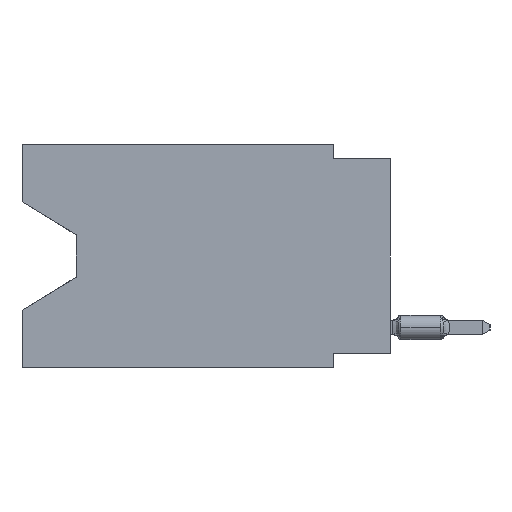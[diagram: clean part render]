
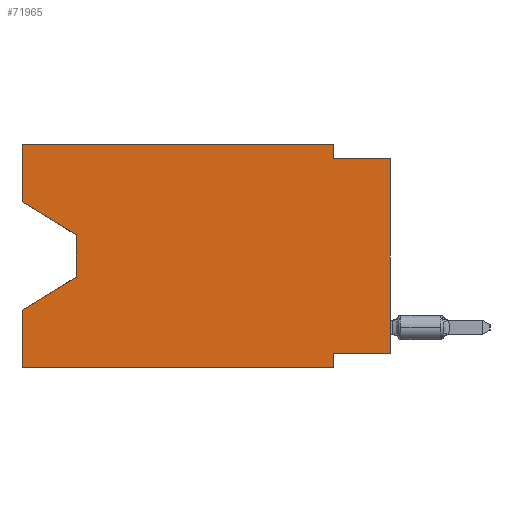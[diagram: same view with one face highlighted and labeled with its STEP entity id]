
A CAD part, left-side view. The second image highlights one B-rep face of the part: STEP entity #71965.
In plain terms, the highlighted planar face has unit normal (-1, 0, 0).
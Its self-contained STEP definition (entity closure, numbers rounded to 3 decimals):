
#1093 = VECTOR ( 'NONE', #67676, 1000. ) ;
#1139 = CARTESIAN_POINT ( 'NONE',  ( 0., 16.383, -2.546 ) ) ;
#1369 = CARTESIAN_POINT ( 'NONE',  ( 0., 13.97, -5.893 ) ) ;
#2217 = LINE ( 'NONE', #28104, #41991 ) ;
#2466 = VERTEX_POINT ( 'NONE', #38149 ) ;
#2677 = DIRECTION ( 'NONE',  ( 0., 0.855, -0.519 ) ) ;
#2856 = ORIENTED_EDGE ( 'NONE', *, *, #49656, .T. ) ;
#4470 = VECTOR ( 'NONE', #2677, 1000. ) ;
#5207 = ORIENTED_EDGE ( 'NONE', *, *, #22602, .T. ) ;
#5239 = ORIENTED_EDGE ( 'NONE', *, *, #23299, .T. ) ;
#5296 = LINE ( 'NONE', #37587, #50493 ) ;
#5646 = CARTESIAN_POINT ( 'NONE',  ( 0., 2.54, -9.906 ) ) ;
#7098 = FACE_OUTER_BOUND ( 'NONE', #19887, .T. ) ;
#7330 = EDGE_CURVE ( 'NONE', #18322, #49611, #44204, .T. ) ;
#7959 = VECTOR ( 'NONE', #17008, 1000. ) ;
#8356 = CARTESIAN_POINT ( 'NONE',  ( 0., 16.383, 0. ) ) ;
#10038 = CARTESIAN_POINT ( 'NONE',  ( 0., 0., -9.271 ) ) ;
#11566 = CARTESIAN_POINT ( 'NONE',  ( 0., 0., -9.271 ) ) ;
#11954 = ORIENTED_EDGE ( 'NONE', *, *, #74613, .F. ) ;
#13325 = EDGE_CURVE ( 'NONE', #49611, #65926, #22198, .T. ) ;
#13948 = CARTESIAN_POINT ( 'NONE',  ( 0., 0., -0.635 ) ) ;
#14406 = ORIENTED_EDGE ( 'NONE', *, *, #48312, .F. ) ;
#15111 = DIRECTION ( 'NONE',  ( 1., 0., 0. ) ) ;
#17008 = DIRECTION ( 'NONE',  ( 0., 0., -1. ) ) ;
#18322 = VERTEX_POINT ( 'NONE', #65536 ) ;
#19887 = EDGE_LOOP ( 'NONE', ( #5239, #55289, #66443, #54813, #5207, #72661, #11954, #2856, #14406, #29574, #67841, #52360 ) ) ;
#20196 = EDGE_CURVE ( 'NONE', #74292, #59708, #28682, .T. ) ;
#20670 = DIRECTION ( 'NONE',  ( 0., -0.855, -0.519 ) ) ;
#22198 = LINE ( 'NONE', #82122, #4470 ) ;
#22303 = DIRECTION ( 'NONE',  ( 0., 0., -1. ) ) ;
#22363 = DIRECTION ( 'NONE',  ( 0., 1., 0. ) ) ;
#22602 = EDGE_CURVE ( 'NONE', #61736, #59708, #33088, .T. ) ;
#23299 = EDGE_CURVE ( 'NONE', #57706, #18322, #39796, .T. ) ;
#24556 = VERTEX_POINT ( 'NONE', #13948 ) ;
#25495 = CARTESIAN_POINT ( 'NONE',  ( 0., 2.54, -9.271 ) ) ;
#26490 = DIRECTION ( 'NONE',  ( 0., -1., 0. ) ) ;
#28104 = CARTESIAN_POINT ( 'NONE',  ( 0., 0., 0. ) ) ;
#28682 = LINE ( 'NONE', #41010, #69854 ) ;
#29574 = ORIENTED_EDGE ( 'NONE', *, *, #31948, .F. ) ;
#31426 = CARTESIAN_POINT ( 'NONE',  ( 0., 13.97, -4.013 ) ) ;
#31948 = EDGE_CURVE ( 'NONE', #51112, #2466, #33709, .T. ) ;
#32020 = EDGE_CURVE ( 'NONE', #61736, #65926, #61739, .T. ) ;
#32816 = CARTESIAN_POINT ( 'NONE',  ( 0., 16.383, -2.546 ) ) ;
#33088 = LINE ( 'NONE', #46265, #62007 ) ;
#33709 = LINE ( 'NONE', #64355, #81165 ) ;
#37587 = CARTESIAN_POINT ( 'NONE',  ( 0., 16.383, 0. ) ) ;
#38065 = EDGE_CURVE ( 'NONE', #57706, #54220, #5296, .T. ) ;
#38149 = CARTESIAN_POINT ( 'NONE',  ( 0., 2.54, -0.635 ) ) ;
#38659 = AXIS2_PLACEMENT_3D ( 'NONE', #8356, #15111, #78914 ) ;
#39198 = CARTESIAN_POINT ( 'NONE',  ( 0., 16.383, -9.906 ) ) ;
#39708 = VECTOR ( 'NONE', #26490, 1000. ) ;
#39793 = PLANE ( 'NONE',  #38659 ) ;
#39796 = LINE ( 'NONE', #1139, #81090 ) ;
#41010 = CARTESIAN_POINT ( 'NONE',  ( 0., 2.54, -9.906 ) ) ;
#41991 = VECTOR ( 'NONE', #54022, 1000. ) ;
#42526 = CARTESIAN_POINT ( 'NONE',  ( 0., 2.54, 0. ) ) ;
#44204 = LINE ( 'NONE', #31426, #7959 ) ;
#44514 = VECTOR ( 'NONE', #22363, 1000. ) ;
#46265 = CARTESIAN_POINT ( 'NONE',  ( 0., 16.383, -9.906 ) ) ;
#46710 = DIRECTION ( 'NONE',  ( 0., -1., 0. ) ) ;
#46730 = VERTEX_POINT ( 'NONE', #11566 ) ;
#48312 = EDGE_CURVE ( 'NONE', #2466, #24556, #70215, .T. ) ;
#49611 = VERTEX_POINT ( 'NONE', #1369 ) ;
#49656 = EDGE_CURVE ( 'NONE', #46730, #24556, #2217, .T. ) ;
#50493 = VECTOR ( 'NONE', #83080, 1000. ) ;
#51112 = VERTEX_POINT ( 'NONE', #42526 ) ;
#52360 = ORIENTED_EDGE ( 'NONE', *, *, #38065, .F. ) ;
#52551 = CARTESIAN_POINT ( 'NONE',  ( 0., 16.383, -7.36 ) ) ;
#53819 = EDGE_CURVE ( 'NONE', #54220, #51112, #71531, .T. ) ;
#54022 = DIRECTION ( 'NONE',  ( 0., 0., 1. ) ) ;
#54220 = VERTEX_POINT ( 'NONE', #71437 ) ;
#54813 = ORIENTED_EDGE ( 'NONE', *, *, #32020, .F. ) ;
#55289 = ORIENTED_EDGE ( 'NONE', *, *, #7330, .T. ) ;
#55330 = CARTESIAN_POINT ( 'NONE',  ( 0., 16.383, 0. ) ) ;
#57706 = VERTEX_POINT ( 'NONE', #32816 ) ;
#57952 = DIRECTION ( 'NONE',  ( 0., 0., -1. ) ) ;
#58778 = CARTESIAN_POINT ( 'NONE',  ( 0., 16.383, 0. ) ) ;
#59025 = DIRECTION ( 'NONE',  ( 0., -1., 0. ) ) ;
#59708 = VERTEX_POINT ( 'NONE', #5646 ) ;
#61736 = VERTEX_POINT ( 'NONE', #39198 ) ;
#61739 = LINE ( 'NONE', #55330, #1093 ) ;
#62007 = VECTOR ( 'NONE', #59025, 1000. ) ;
#63838 = CARTESIAN_POINT ( 'NONE',  ( 0., 0., -0.635 ) ) ;
#64355 = CARTESIAN_POINT ( 'NONE',  ( 0., 2.54, 0. ) ) ;
#65536 = CARTESIAN_POINT ( 'NONE',  ( 0., 13.97, -4.013 ) ) ;
#65926 = VERTEX_POINT ( 'NONE', #52551 ) ;
#66443 = ORIENTED_EDGE ( 'NONE', *, *, #13325, .T. ) ;
#67676 = DIRECTION ( 'NONE',  ( 0., 0., 1. ) ) ;
#67841 = ORIENTED_EDGE ( 'NONE', *, *, #53819, .F. ) ;
#68249 = LINE ( 'NONE', #10038, #44514 ) ;
#69854 = VECTOR ( 'NONE', #22303, 1000. ) ;
#70215 = LINE ( 'NONE', #63838, #73280 ) ;
#71437 = CARTESIAN_POINT ( 'NONE',  ( 0., 16.383, 0. ) ) ;
#71531 = LINE ( 'NONE', #58778, #39708 ) ;
#71965 = ADVANCED_FACE ( 'NONE', ( #7098 ), #39793, .F. ) ;
#72661 = ORIENTED_EDGE ( 'NONE', *, *, #20196, .F. ) ;
#73280 = VECTOR ( 'NONE', #46710, 1000. ) ;
#74292 = VERTEX_POINT ( 'NONE', #25495 ) ;
#74613 = EDGE_CURVE ( 'NONE', #46730, #74292, #68249, .T. ) ;
#78914 = DIRECTION ( 'NONE',  ( 0., 0., -1. ) ) ;
#81090 = VECTOR ( 'NONE', #20670, 1000. ) ;
#81165 = VECTOR ( 'NONE', #57952, 1000. ) ;
#82122 = CARTESIAN_POINT ( 'NONE',  ( 0., 13.97, -5.893 ) ) ;
#83080 = DIRECTION ( 'NONE',  ( 0., 0., 1. ) ) ;
